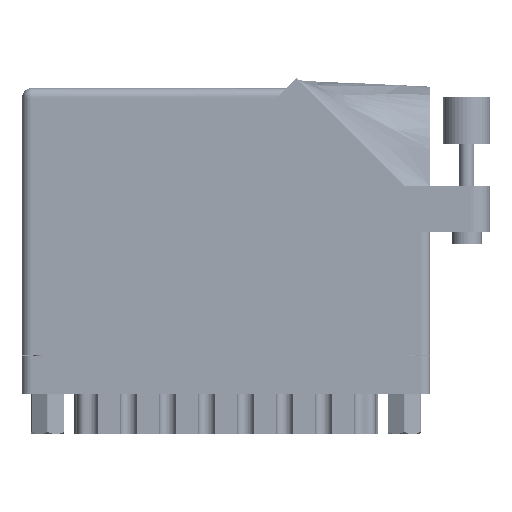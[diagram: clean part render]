
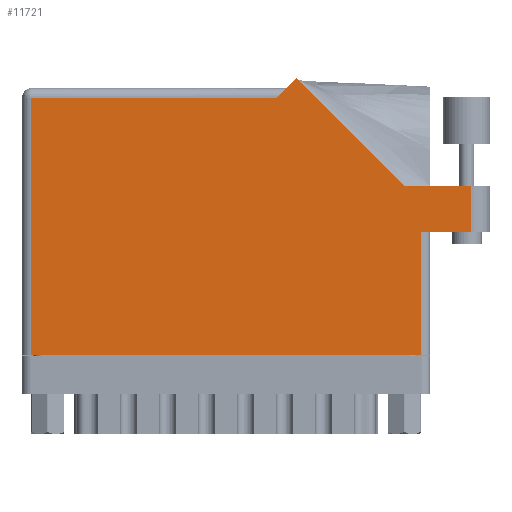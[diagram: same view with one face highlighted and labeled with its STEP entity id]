
A CAD part, front view. The second image highlights one B-rep face of the part: STEP entity #11721.
In plain terms, the highlighted face is planar.
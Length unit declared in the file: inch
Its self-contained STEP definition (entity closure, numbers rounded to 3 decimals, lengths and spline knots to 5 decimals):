
#1259 = ORIENTED_EDGE ( 'NONE', *, *, #48127, .T. ) ;
#1611 = DIRECTION ( 'NONE',  ( -1., 0., 0. ) ) ;
#4185 = EDGE_LOOP ( 'NONE', ( #63806, #26566, #21468, #5029, #11445, #45279, #54144, #19553, #1259 ) ) ;
#5029 = ORIENTED_EDGE ( 'NONE', *, *, #75213, .T. ) ;
#5208 = VERTEX_POINT ( 'NONE', #14050 ) ;
#5631 = DIRECTION ( 'NONE',  ( 1., 0., 0. ) ) ;
#6576 = LINE ( 'NONE', #52867, #75199 ) ;
#7732 = EDGE_CURVE ( 'NONE', #57688, #37769, #71793, .T. ) ;
#7909 = LINE ( 'NONE', #65428, #65122 ) ;
#8855 = VECTOR ( 'NONE', #25634, 39.37008 ) ;
#9852 = CARTESIAN_POINT ( 'NONE',  ( 2.993, 1.122, 0. ) ) ;
#10435 = EDGE_CURVE ( 'NONE', #58662, #57688, #49955, .T. ) ;
#11052 = CARTESIAN_POINT ( 'NONE',  ( 0., 0., 0. ) ) ;
#11223 = VECTOR ( 'NONE', #18915, 39.37008 ) ;
#11417 = CARTESIAN_POINT ( 'NONE',  ( 2.718, 0.815, 0. ) ) ;
#11445 = ORIENTED_EDGE ( 'NONE', *, *, #30232, .T. ) ;
#11721 = ADVANCED_FACE ( 'NONE', ( #22705 ), #41992, .F. ) ;
#12128 = VERTEX_POINT ( 'NONE', #39867 ) ;
#14022 = LINE ( 'NONE', #11417, #45237 ) ;
#14050 = CARTESIAN_POINT ( 'NONE',  ( 0.062, 0., 0. ) ) ;
#14233 = LINE ( 'NONE', #48781, #23581 ) ;
#14388 = DIRECTION ( 'NONE',  ( -1., 0., 0. ) ) ;
#16514 = EDGE_CURVE ( 'NONE', #47270, #58662, #14022, .T. ) ;
#17715 = VECTOR ( 'NONE', #46527, 39.37008 ) ;
#18293 = CARTESIAN_POINT ( 'NONE',  ( 1.82871, 1.84571, 0. ) ) ;
#18915 = DIRECTION ( 'NONE',  ( -1., 0., 0. ) ) ;
#19553 = ORIENTED_EDGE ( 'NONE', *, *, #52128, .T. ) ;
#21468 = ORIENTED_EDGE ( 'NONE', *, *, #7732, .T. ) ;
#22705 = FACE_OUTER_BOUND ( 'NONE', #4185, .T. ) ;
#23123 = VERTEX_POINT ( 'NONE', #37467 ) ;
#23581 = VECTOR ( 'NONE', #35985, 39.37008 ) ;
#25634 = DIRECTION ( 'NONE',  ( -0.707, -0.707, 0. ) ) ;
#26369 = CARTESIAN_POINT ( 'NONE',  ( 0.062, 1.713, 0. ) ) ;
#26402 = DIRECTION ( 'NONE',  ( -0.707, 0.707, 0. ) ) ;
#26547 = LINE ( 'NONE', #71526, #8855 ) ;
#26566 = ORIENTED_EDGE ( 'NONE', *, *, #10435, .T. ) ;
#26756 = CARTESIAN_POINT ( 'NONE',  ( 0., 1.713, 0. ) ) ;
#30232 = EDGE_CURVE ( 'NONE', #85932, #23123, #26547, .T. ) ;
#31157 = DIRECTION ( 'NONE',  ( 1., 0., 0. ) ) ;
#33789 = CARTESIAN_POINT ( 'NONE',  ( 2.656, 0.815, 0. ) ) ;
#34414 = VECTOR ( 'NONE', #14388, 39.37008 ) ;
#35985 = DIRECTION ( 'NONE',  ( 0., 1., 0. ) ) ;
#36244 = VERTEX_POINT ( 'NONE', #26369 ) ;
#37467 = CARTESIAN_POINT ( 'NONE',  ( 1.696, 1.713, 0. ) ) ;
#37769 = VERTEX_POINT ( 'NONE', #44456 ) ;
#38999 = EDGE_CURVE ( 'NONE', #23123, #36244, #49753, .T. ) ;
#39867 = CARTESIAN_POINT ( 'NONE',  ( 2.656, 0., 0. ) ) ;
#41992 = PLANE ( 'NONE',  #82538 ) ;
#44456 = CARTESIAN_POINT ( 'NONE',  ( 2.55242, 1.122, 0. ) ) ;
#45237 = VECTOR ( 'NONE', #5631, 39.37008 ) ;
#45279 = ORIENTED_EDGE ( 'NONE', *, *, #38999, .T. ) ;
#46527 = DIRECTION ( 'NONE',  ( 0., 1., 0. ) ) ;
#47270 = VERTEX_POINT ( 'NONE', #33789 ) ;
#48127 = EDGE_CURVE ( 'NONE', #12128, #47270, #14233, .T. ) ;
#48781 = CARTESIAN_POINT ( 'NONE',  ( 2.656, 0.815, 0. ) ) ;
#49753 = LINE ( 'NONE', #26756, #11223 ) ;
#49955 = LINE ( 'NONE', #72087, #17715 ) ;
#52128 = EDGE_CURVE ( 'NONE', #5208, #12128, #67154, .T. ) ;
#52867 = CARTESIAN_POINT ( 'NONE',  ( 2.55242, 1.122, 0. ) ) ;
#54144 = ORIENTED_EDGE ( 'NONE', *, *, #60516, .T. ) ;
#54244 = CARTESIAN_POINT ( 'NONE',  ( 3.118, 1.122, 0. ) ) ;
#55075 = CARTESIAN_POINT ( 'NONE',  ( 0., 1.775, 0. ) ) ;
#57688 = VERTEX_POINT ( 'NONE', #9852 ) ;
#58662 = VERTEX_POINT ( 'NONE', #85118 ) ;
#60516 = EDGE_CURVE ( 'NONE', #36244, #5208, #7909, .T. ) ;
#61748 = DIRECTION ( 'NONE',  ( 0., 0., -1. ) ) ;
#63806 = ORIENTED_EDGE ( 'NONE', *, *, #16514, .T. ) ;
#65122 = VECTOR ( 'NONE', #65713, 39.37008 ) ;
#65428 = CARTESIAN_POINT ( 'NONE',  ( 0.062, 0., 0. ) ) ;
#65713 = DIRECTION ( 'NONE',  ( 0., -1., 0. ) ) ;
#67154 = LINE ( 'NONE', #11052, #84800 ) ;
#71526 = CARTESIAN_POINT ( 'NONE',  ( 1.758, 1.775, 0. ) ) ;
#71793 = LINE ( 'NONE', #54244, #34414 ) ;
#72087 = CARTESIAN_POINT ( 'NONE',  ( 2.993, 1.122, 0. ) ) ;
#75199 = VECTOR ( 'NONE', #26402, 39.37008 ) ;
#75213 = EDGE_CURVE ( 'NONE', #37769, #85932, #6576, .T. ) ;
#82538 = AXIS2_PLACEMENT_3D ( 'NONE', #55075, #61748, #1611 ) ;
#84800 = VECTOR ( 'NONE', #31157, 39.37008 ) ;
#85118 = CARTESIAN_POINT ( 'NONE',  ( 2.993, 0.815, 0. ) ) ;
#85932 = VERTEX_POINT ( 'NONE', #18293 ) ;
